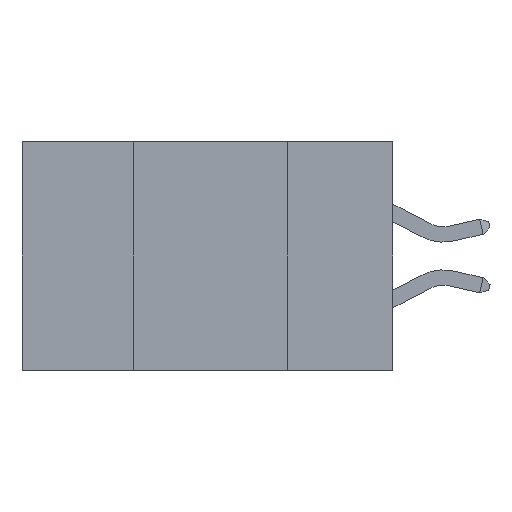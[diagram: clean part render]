
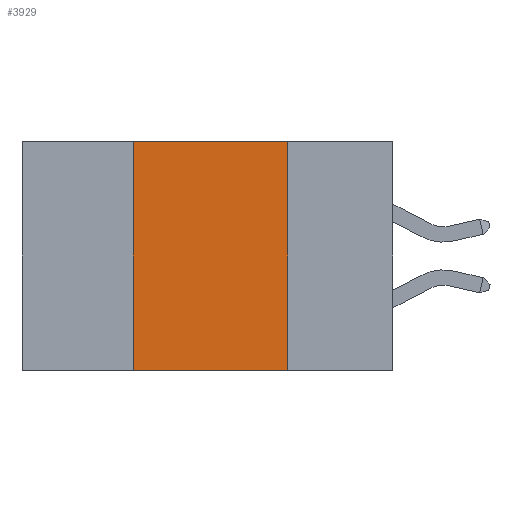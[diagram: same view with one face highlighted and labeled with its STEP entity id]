
A CAD part, left-side view. The second image highlights one B-rep face of the part: STEP entity #3929.
In plain terms, the highlighted planar face has unit normal (-1, 0, 0).
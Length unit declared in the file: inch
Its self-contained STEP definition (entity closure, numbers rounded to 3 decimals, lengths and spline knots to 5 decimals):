
#145 = FACE_OUTER_BOUND ( 'NONE', #19433, .T. ) ;
#261 = CARTESIAN_POINT ( 'NONE',  ( 0., 0.6, 0. ) ) ;
#555 = DIRECTION ( 'NONE',  ( 0., -1., 0. ) ) ;
#835 = VERTEX_POINT ( 'NONE', #10768 ) ;
#1414 = EDGE_CURVE ( 'NONE', #835, #11971, #12821, .T. ) ;
#3233 = ORIENTED_EDGE ( 'NONE', *, *, #16258, .T. ) ;
#3557 = PLANE ( 'NONE',  #11268 ) ;
#3606 = CARTESIAN_POINT ( 'NONE',  ( 0., 0.42, 0. ) ) ;
#3929 = ADVANCED_FACE ( 'NONE', ( #145 ), #3557, .F. ) ;
#4036 = VECTOR ( 'NONE', #18734, 39.37008 ) ;
#5157 = DIRECTION ( 'NONE',  ( 0., 0., -1. ) ) ;
#6689 = VECTOR ( 'NONE', #555, 39.37008 ) ;
#7113 = VECTOR ( 'NONE', #12864, 39.37008 ) ;
#8718 = LINE ( 'NONE', #9524, #4036 ) ;
#8783 = VECTOR ( 'NONE', #18664, 39.37008 ) ;
#9007 = VERTEX_POINT ( 'NONE', #3606 ) ;
#9524 = CARTESIAN_POINT ( 'NONE',  ( 0., 0.6, -0.37 ) ) ;
#10093 = CARTESIAN_POINT ( 'NONE',  ( 0., 0.6, 0. ) ) ;
#10321 = LINE ( 'NONE', #10093, #6689 ) ;
#10768 = CARTESIAN_POINT ( 'NONE',  ( 0., 0.17, 0. ) ) ;
#11077 = ORIENTED_EDGE ( 'NONE', *, *, #12575, .F. ) ;
#11234 = LINE ( 'NONE', #19021, #7113 ) ;
#11268 = AXIS2_PLACEMENT_3D ( 'NONE', #261, #14430, #5157 ) ;
#11780 = CARTESIAN_POINT ( 'NONE',  ( 0., 0.17, -0.37 ) ) ;
#11887 = VERTEX_POINT ( 'NONE', #13034 ) ;
#11971 = VERTEX_POINT ( 'NONE', #11780 ) ;
#12575 = EDGE_CURVE ( 'NONE', #9007, #835, #10321, .T. ) ;
#12821 = LINE ( 'NONE', #17154, #8783 ) ;
#12864 = DIRECTION ( 'NONE',  ( 0., 0., 1. ) ) ;
#13034 = CARTESIAN_POINT ( 'NONE',  ( 0., 0.42, -0.37 ) ) ;
#14430 = DIRECTION ( 'NONE',  ( 1., 0., 0. ) ) ;
#15181 = ORIENTED_EDGE ( 'NONE', *, *, #19285, .F. ) ;
#16258 = EDGE_CURVE ( 'NONE', #11887, #11971, #8718, .T. ) ;
#17154 = CARTESIAN_POINT ( 'NONE',  ( 0., 0.17, 0. ) ) ;
#18664 = DIRECTION ( 'NONE',  ( 0., 0., -1. ) ) ;
#18734 = DIRECTION ( 'NONE',  ( 0., -1., 0. ) ) ;
#18770 = ORIENTED_EDGE ( 'NONE', *, *, #1414, .F. ) ;
#19021 = CARTESIAN_POINT ( 'NONE',  ( 0., 0.42, 0. ) ) ;
#19285 = EDGE_CURVE ( 'NONE', #11887, #9007, #11234, .T. ) ;
#19433 = EDGE_LOOP ( 'NONE', ( #18770, #11077, #15181, #3233 ) ) ;
